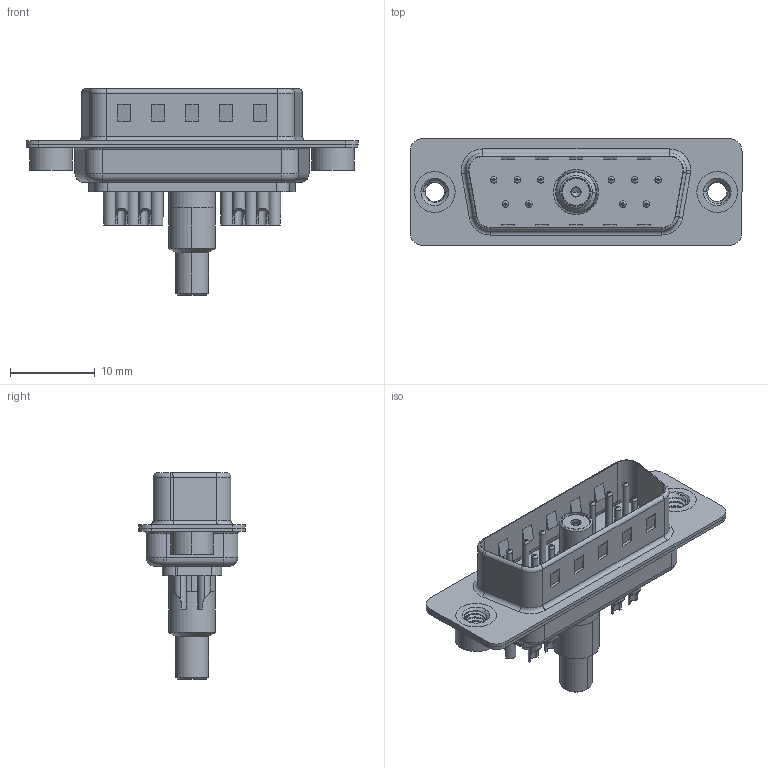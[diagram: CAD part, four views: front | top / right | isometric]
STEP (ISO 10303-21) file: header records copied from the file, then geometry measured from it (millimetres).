
FILE_DESCRIPTION (( 'STEP AP203' ), '1' );
FILE_NAME ('627-11W1622-7TA.STEP', '2019-05-25T15:01:40', ( '' ), ( '' ), 'SwSTEP 2.0', 'SolidWorks 2016', '' );
FILE_SCHEMA (( 'CONFIG_CONTROL_DESIGN' ));
Length unit declared in the file: millimetre
Products named in the file (15): Co-Ax Jack Assy_SC; 627Combo Shell Front_15 Contacts; 627Combo Threaded Rivet_2; 627Combo Threaded Rivet_A; 627Combo Contact Row 1_22; Co-Ax Jack_Solder Cup Tail; 627Combo Contact Row 2_22; Insulator Socket; 627-11W1622-7TA; Insulator Socket 2; Locking Collar; Socket_Solder Cup; 627Combo Housing_11W1; Solder Cover; 627Combo Shell Rear_15 Contacts
Assembly tree (22 placements, depth 3):
  627-11W1622-7TA
    627Combo Housing_11W1
    627Combo Shell Rear_15 Contacts
    627Combo Shell Front_15 Contacts
    627Combo Threaded Rivet_A
    Co-Ax Jack Assy_SC
      Co-Ax Jack_Solder Cup Tail
      Insulator Socket
      Insulator Socket 2
      Locking Collar
      Socket_Solder Cup
      Solder Cover
    627Combo Threaded Rivet_2
    627Combo Contact Row 1_22  x6
    627Combo Contact Row 2_22  x4
Bounding box: 39.15 x 12.6 x 24.3 mm (x, y, z)
Volume: 1986.2 mm3; surface area: 5703.8 mm2
Topology: 21 solids, 24 shells, 852 faces, 2004 edges, 1236 vertices
Faces by surface type: cylinder 362, plane 278, torus 154, cone 50, bspline 8
Entity records: 23123 total; most frequent: CARTESIAN_POINT 6578, DIRECTION 3282, ORIENTED_EDGE 2932, EDGE_CURVE 1466, AXIS2_PLACEMENT_3D 1291, VERTEX_POINT 924, EDGE_LOOP 734, VECTOR 700
